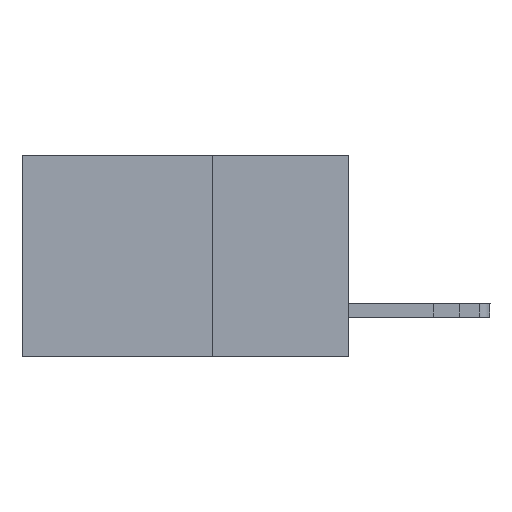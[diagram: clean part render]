
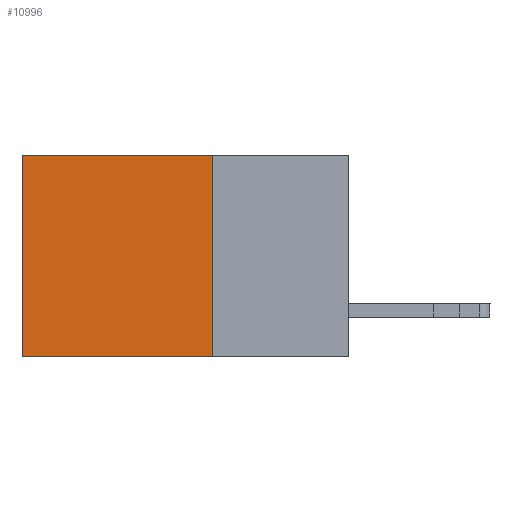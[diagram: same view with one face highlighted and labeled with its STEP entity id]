
A CAD part, left-side view. The second image highlights one B-rep face of the part: STEP entity #10996.
In plain terms, the highlighted planar face has unit normal (-1, 0, 0).
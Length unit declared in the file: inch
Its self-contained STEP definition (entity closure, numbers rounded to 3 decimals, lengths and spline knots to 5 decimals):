
#786 = EDGE_CURVE ( 'NONE', #19972, #1995, #18274, .T. ) ;
#854 = VECTOR ( 'NONE', #13631, 39.37008 ) ;
#1411 = VERTEX_POINT ( 'NONE', #19717 ) ;
#1980 = DIRECTION ( 'NONE',  ( 0., 0., -1. ) ) ;
#1995 = VERTEX_POINT ( 'NONE', #14857 ) ;
#2189 = DIRECTION ( 'NONE',  ( 0., 0., -1. ) ) ;
#3562 = CARTESIAN_POINT ( 'NONE',  ( 0.2615, 0.6, 0. ) ) ;
#3767 = CARTESIAN_POINT ( 'NONE',  ( 0.2615, 0.25, -0.37 ) ) ;
#4925 = ORIENTED_EDGE ( 'NONE', *, *, #14208, .F. ) ;
#5072 = LINE ( 'NONE', #12016, #854 ) ;
#5564 = LINE ( 'NONE', #3767, #17855 ) ;
#5914 = CARTESIAN_POINT ( 'NONE',  ( 0.2615, 0.25, 0. ) ) ;
#6118 = ORIENTED_EDGE ( 'NONE', *, *, #16153, .F. ) ;
#9756 = VECTOR ( 'NONE', #13998, 39.37008 ) ;
#9948 = PLANE ( 'NONE',  #13182 ) ;
#10693 = ORIENTED_EDGE ( 'NONE', *, *, #19238, .T. ) ;
#10996 = ADVANCED_FACE ( 'NONE', ( #14959 ), #9948, .F. ) ;
#11567 = DIRECTION ( 'NONE',  ( 1., 0., 0. ) ) ;
#12016 = CARTESIAN_POINT ( 'NONE',  ( 0.2615, 0.25, -0.37 ) ) ;
#13182 = AXIS2_PLACEMENT_3D ( 'NONE', #14692, #11567, #1980 ) ;
#13631 = DIRECTION ( 'NONE',  ( 0., 1., 0. ) ) ;
#13848 = CARTESIAN_POINT ( 'NONE',  ( 0.2615, 0.25, -0.37 ) ) ;
#13998 = DIRECTION ( 'NONE',  ( 0., 1., 0. ) ) ;
#14208 = EDGE_CURVE ( 'NONE', #1411, #17841, #5564, .T. ) ;
#14692 = CARTESIAN_POINT ( 'NONE',  ( 0.2615, 0.25, -0.37 ) ) ;
#14857 = CARTESIAN_POINT ( 'NONE',  ( 0.2615, 0.6, -0.37 ) ) ;
#14959 = FACE_OUTER_BOUND ( 'NONE', #19150, .T. ) ;
#16153 = EDGE_CURVE ( 'NONE', #17841, #1995, #5072, .T. ) ;
#17841 = VERTEX_POINT ( 'NONE', #13848 ) ;
#17855 = VECTOR ( 'NONE', #2189, 39.37008 ) ;
#18274 = LINE ( 'NONE', #19694, #18773 ) ;
#18747 = LINE ( 'NONE', #5914, #9756 ) ;
#18773 = VECTOR ( 'NONE', #19329, 39.37008 ) ;
#19150 = EDGE_LOOP ( 'NONE', ( #19303, #6118, #4925, #10693 ) ) ;
#19238 = EDGE_CURVE ( 'NONE', #1411, #19972, #18747, .T. ) ;
#19303 = ORIENTED_EDGE ( 'NONE', *, *, #786, .T. ) ;
#19329 = DIRECTION ( 'NONE',  ( 0., 0., -1. ) ) ;
#19694 = CARTESIAN_POINT ( 'NONE',  ( 0.2615, 0.6, -0.37 ) ) ;
#19717 = CARTESIAN_POINT ( 'NONE',  ( 0.2615, 0.25, 0. ) ) ;
#19972 = VERTEX_POINT ( 'NONE', #3562 ) ;
